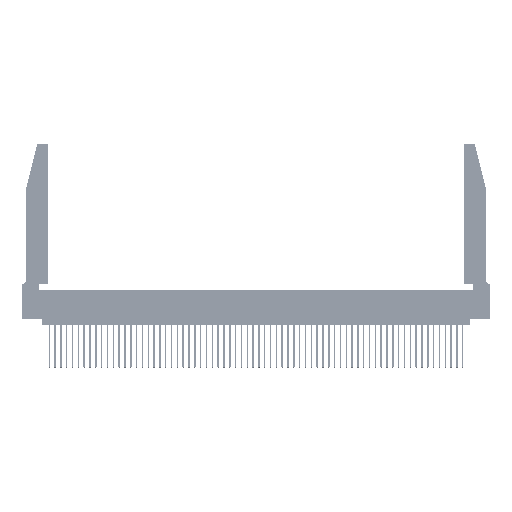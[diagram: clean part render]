
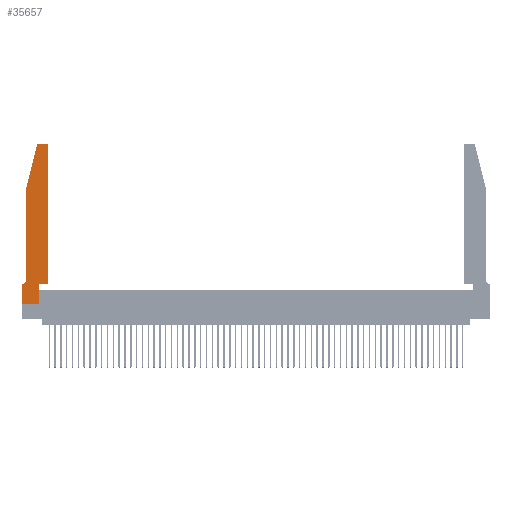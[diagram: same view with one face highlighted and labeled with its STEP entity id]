
A CAD part, top view. The second image highlights one B-rep face of the part: STEP entity #35657.
In plain terms, the highlighted planar face has unit normal (0, 0, 1).
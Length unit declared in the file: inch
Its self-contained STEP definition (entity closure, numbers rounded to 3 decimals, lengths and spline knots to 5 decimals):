
#479 = CARTESIAN_POINT ( 'NONE',  ( 0.0755, 2., 0.37 ) ) ;
#1048 = VERTEX_POINT ( 'NONE', #49388 ) ;
#2592 = CARTESIAN_POINT ( 'NONE',  ( 0.0755, 0.42, 0.37 ) ) ;
#3156 = EDGE_CURVE ( 'NONE', #32051, #23126, #38475, .T. ) ;
#4176 = CARTESIAN_POINT ( 'NONE',  ( 0.4205, 2.75, 0.37 ) ) ;
#5159 = CARTESIAN_POINT ( 'NONE',  ( 0.4505, 0.35, 0.37 ) ) ;
#5476 = VECTOR ( 'NONE', #50119, 39.37008 ) ;
#5595 = DIRECTION ( 'NONE',  ( 0., 0., 1. ) ) ;
#5782 = VERTEX_POINT ( 'NONE', #4176 ) ;
#6075 = AXIS2_PLACEMENT_3D ( 'NONE', #46343, #24063, #11122 ) ;
#7486 = AXIS2_PLACEMENT_3D ( 'NONE', #35813, #22238, #17586 ) ;
#7540 = ORIENTED_EDGE ( 'NONE', *, *, #20704, .T. ) ;
#8144 = EDGE_CURVE ( 'NONE', #36024, #43510, #32102, .T. ) ;
#8528 = AXIS2_PLACEMENT_3D ( 'NONE', #30472, #21916, #18429 ) ;
#9077 = EDGE_LOOP ( 'NONE', ( #24866, #17403, #7540, #47037, #41926, #32301, #37436, #10334, #48377, #50140, #16255, #38764 ) ) ;
#9646 = DIRECTION ( 'NONE',  ( 1., 0., 0. ) ) ;
#10068 = CARTESIAN_POINT ( 'NONE',  ( 0.0055, 0.35, 0.37 ) ) ;
#10334 = ORIENTED_EDGE ( 'NONE', *, *, #37592, .T. ) ;
#11122 = DIRECTION ( 'NONE',  ( 1., 0., 0. ) ) ;
#11238 = CARTESIAN_POINT ( 'NONE',  ( 0.2865, 0.35, 0.37 ) ) ;
#12800 = CIRCLE ( 'NONE', #7486, 0.07 ) ;
#14163 = FACE_OUTER_BOUND ( 'NONE', #9077, .T. ) ;
#14890 = CARTESIAN_POINT ( 'NONE',  ( 0., 0., 0.37 ) ) ;
#16255 = ORIENTED_EDGE ( 'NONE', *, *, #3156, .T. ) ;
#16693 = EDGE_CURVE ( 'NONE', #23126, #5782, #26959, .T. ) ;
#16718 = CARTESIAN_POINT ( 'NONE',  ( 0.4505, 0.35, 0.37 ) ) ;
#16998 = LINE ( 'NONE', #46970, #30948 ) ;
#17403 = ORIENTED_EDGE ( 'NONE', *, *, #8144, .T. ) ;
#17507 = DIRECTION ( 'NONE',  ( 0., -1., 0. ) ) ;
#17586 = DIRECTION ( 'NONE',  ( -1., 0., 0. ) ) ;
#18429 = DIRECTION ( 'NONE',  ( 1., 0., 0. ) ) ;
#19323 = LINE ( 'NONE', #14890, #5476 ) ;
#20358 = AXIS2_PLACEMENT_3D ( 'NONE', #27096, #5595, #27484 ) ;
#20704 = EDGE_CURVE ( 'NONE', #43510, #1048, #39772, .T. ) ;
#21916 = DIRECTION ( 'NONE',  ( 0., 0., 1. ) ) ;
#22238 = DIRECTION ( 'NONE',  ( 0., 0., -1. ) ) ;
#23126 = VERTEX_POINT ( 'NONE', #53816 ) ;
#23192 = LINE ( 'NONE', #56916, #35732 ) ;
#23816 = VECTOR ( 'NONE', #33148, 39.37008 ) ;
#24063 = DIRECTION ( 'NONE',  ( 0., 0., 1. ) ) ;
#24092 = VECTOR ( 'NONE', #9646, 39.37008 ) ;
#24121 = VERTEX_POINT ( 'NONE', #2592 ) ;
#24473 = VECTOR ( 'NONE', #34891, 39.37008 ) ;
#24866 = ORIENTED_EDGE ( 'NONE', *, *, #41522, .T. ) ;
#25260 = EDGE_CURVE ( 'NONE', #54209, #32051, #51176, .T. ) ;
#26497 = CARTESIAN_POINT ( 'NONE',  ( 0., 0.35, 0.37 ) ) ;
#26959 = CIRCLE ( 'NONE', #6075, 0.03 ) ;
#27096 = CARTESIAN_POINT ( 'NONE',  ( 0.284, 2.72, 0.37 ) ) ;
#27484 = DIRECTION ( 'NONE',  ( 1., 0., 0. ) ) ;
#27574 = DIRECTION ( 'NONE',  ( 0., 1., 0. ) ) ;
#30260 = LINE ( 'NONE', #49287, #37197 ) ;
#30472 = CARTESIAN_POINT ( 'NONE',  ( 0., 0.35, 0.37 ) ) ;
#30948 = VECTOR ( 'NONE', #51056, 39.37008 ) ;
#31618 = VECTOR ( 'NONE', #17507, 39.37008 ) ;
#32051 = VERTEX_POINT ( 'NONE', #16718 ) ;
#32102 = CIRCLE ( 'NONE', #20358, 0.03 ) ;
#32301 = ORIENTED_EDGE ( 'NONE', *, *, #34832, .T. ) ;
#33001 = DIRECTION ( 'NONE',  ( -0.239, -0.971, 0. ) ) ;
#33148 = DIRECTION ( 'NONE',  ( 0., 1., 0. ) ) ;
#34832 = EDGE_CURVE ( 'NONE', #41893, #39271, #16998, .T. ) ;
#34891 = DIRECTION ( 'NONE',  ( -1., 0., 0. ) ) ;
#35084 = EDGE_CURVE ( 'NONE', #1048, #24121, #43337, .T. ) ;
#35657 = ADVANCED_FACE ( 'NONE', ( #14163 ), #36247, .T. ) ;
#35732 = VECTOR ( 'NONE', #43339, 39.37008 ) ;
#35813 = CARTESIAN_POINT ( 'NONE',  ( 0.0055, 0.42, 0.37 ) ) ;
#36024 = VERTEX_POINT ( 'NONE', #56370 ) ;
#36247 = PLANE ( 'NONE',  #8528 ) ;
#36300 = LINE ( 'NONE', #57151, #24473 ) ;
#36663 = CARTESIAN_POINT ( 'NONE',  ( 0., 0., 0.37 ) ) ;
#37197 = VECTOR ( 'NONE', #27574, 39.37008 ) ;
#37436 = ORIENTED_EDGE ( 'NONE', *, *, #44961, .T. ) ;
#37592 = EDGE_CURVE ( 'NONE', #44254, #50254, #19323, .T. ) ;
#37621 = CARTESIAN_POINT ( 'NONE',  ( 0.0755, 2., 0.37 ) ) ;
#38380 = VECTOR ( 'NONE', #33001, 39.37008 ) ;
#38475 = LINE ( 'NONE', #46643, #23816 ) ;
#38764 = ORIENTED_EDGE ( 'NONE', *, *, #16693, .T. ) ;
#39271 = VERTEX_POINT ( 'NONE', #26497 ) ;
#39772 = LINE ( 'NONE', #37621, #38380 ) ;
#40057 = EDGE_CURVE ( 'NONE', #50254, #54209, #30260, .T. ) ;
#40963 = CARTESIAN_POINT ( 'NONE',  ( 0.25487, 2.72718, 0.37 ) ) ;
#41522 = EDGE_CURVE ( 'NONE', #5782, #36024, #36300, .T. ) ;
#41893 = VERTEX_POINT ( 'NONE', #10068 ) ;
#41926 = ORIENTED_EDGE ( 'NONE', *, *, #52620, .T. ) ;
#43337 = LINE ( 'NONE', #479, #31618 ) ;
#43339 = DIRECTION ( 'NONE',  ( 0., -1., 0. ) ) ;
#43510 = VERTEX_POINT ( 'NONE', #40963 ) ;
#44254 = VERTEX_POINT ( 'NONE', #36663 ) ;
#44961 = EDGE_CURVE ( 'NONE', #39271, #44254, #23192, .T. ) ;
#46343 = CARTESIAN_POINT ( 'NONE',  ( 0.4205, 2.72, 0.37 ) ) ;
#46643 = CARTESIAN_POINT ( 'NONE',  ( 0.4505, 0.35, 0.37 ) ) ;
#46970 = CARTESIAN_POINT ( 'NONE',  ( 0.0755, 0.35, 0.37 ) ) ;
#47037 = ORIENTED_EDGE ( 'NONE', *, *, #35084, .T. ) ;
#48377 = ORIENTED_EDGE ( 'NONE', *, *, #40057, .T. ) ;
#49287 = CARTESIAN_POINT ( 'NONE',  ( 0.2865, 0.35, 0.37 ) ) ;
#49388 = CARTESIAN_POINT ( 'NONE',  ( 0.0755, 2., 0.37 ) ) ;
#49810 = CARTESIAN_POINT ( 'NONE',  ( 0.2865, 0., 0.37 ) ) ;
#50119 = DIRECTION ( 'NONE',  ( 1., 0., 0. ) ) ;
#50140 = ORIENTED_EDGE ( 'NONE', *, *, #25260, .T. ) ;
#50254 = VERTEX_POINT ( 'NONE', #49810 ) ;
#51056 = DIRECTION ( 'NONE',  ( -1., 0., 0. ) ) ;
#51176 = LINE ( 'NONE', #5159, #24092 ) ;
#52620 = EDGE_CURVE ( 'NONE', #24121, #41893, #12800, .T. ) ;
#53816 = CARTESIAN_POINT ( 'NONE',  ( 0.4505, 2.72, 0.37 ) ) ;
#54209 = VERTEX_POINT ( 'NONE', #11238 ) ;
#56370 = CARTESIAN_POINT ( 'NONE',  ( 0.284, 2.75, 0.37 ) ) ;
#56916 = CARTESIAN_POINT ( 'NONE',  ( 0., 0., 0.37 ) ) ;
#57151 = CARTESIAN_POINT ( 'NONE',  ( 0.2605, 2.75, 0.37 ) ) ;
